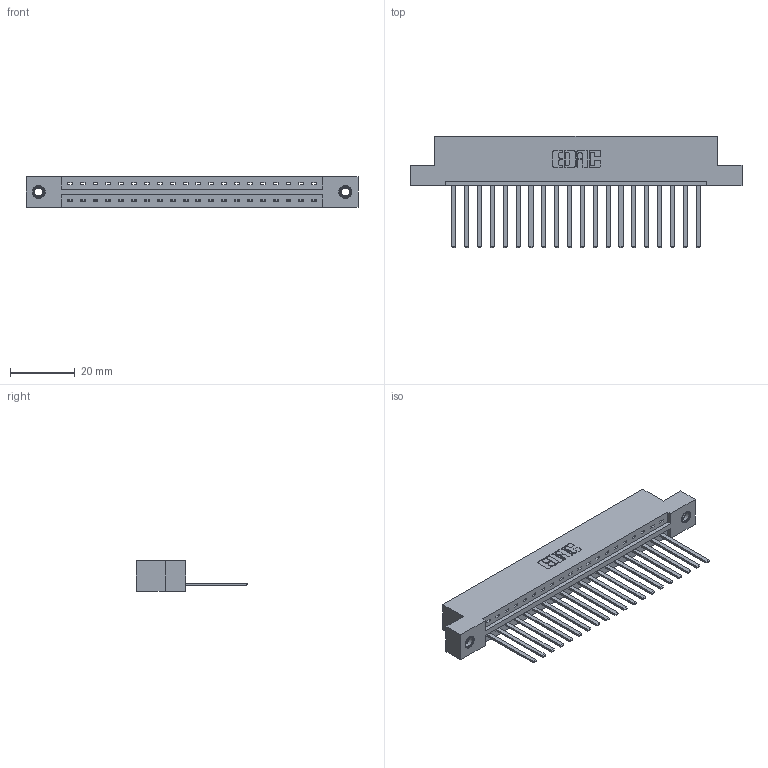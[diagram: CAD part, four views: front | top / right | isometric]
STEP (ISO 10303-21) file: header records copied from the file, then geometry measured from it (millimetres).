
FILE_DESCRIPTION (( 'STEP AP203' ), '1' );
FILE_NAME ('387-020-544-107.STEP', '2019-10-02T23:01:51', ( '' ), ( '' ), 'SwSTEP 2.0', 'SolidWorks 2016', '' );
FILE_SCHEMA (( 'CONFIG_CONTROL_DESIGN' ));
Length unit declared in the file: inch
Products named in the file (4): 345-292-001_345-293-144; 387-020-544-107; 337 Part_Flush Mounting Lugs - 0.156 Dia-TI; 345-250-001_345-250-005-103
Assembly tree (23 placements, depth 2):
  387-020-544-107
    337 Part_Flush Mounting Lugs - 0.156 Dia-TI
    345-292-001_345-293-144  x20
    345-250-001_345-250-005-103  x2
Bounding box: 102.26 x 34.3 x 9.4 mm (x, y, z)
Volume: 10571.1 mm3; surface area: 11604.5 mm2
Topology: 23 solids, 23 shells, 1294 faces, 3847 edges, 2530 vertices
Faces by surface type: plane 942, cylinder 336, cone 12, torus 4
Entity records: 18714 total; most frequent: CARTESIAN_POINT 3237, ORIENTED_EDGE 3186, DIRECTION 2799, EDGE_CURVE 1593, LINE 1449, VECTOR 1449, VERTEX_POINT 1056, AXIS2_PLACEMENT_3D 675
